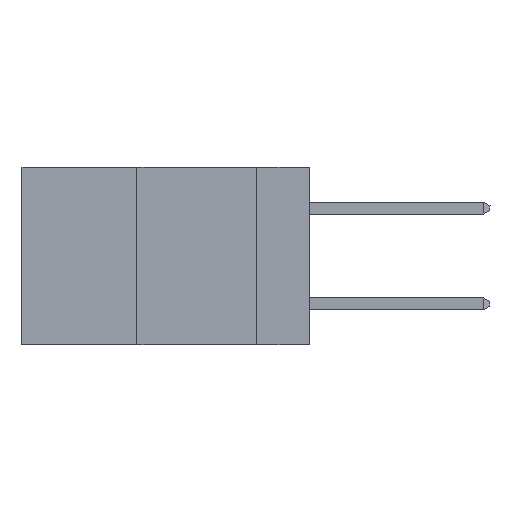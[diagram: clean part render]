
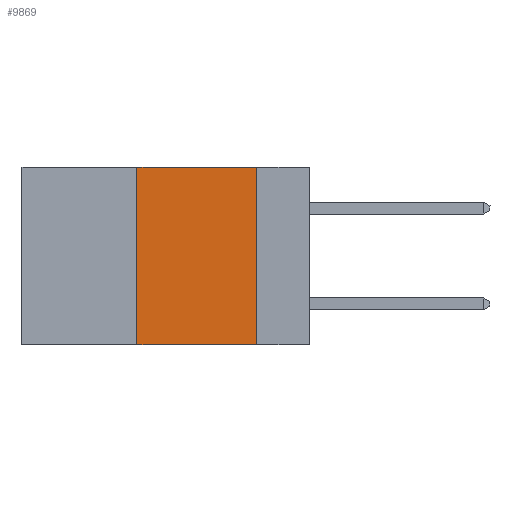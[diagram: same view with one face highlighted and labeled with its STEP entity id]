
A CAD part, left-side view. The second image highlights one B-rep face of the part: STEP entity #9869.
In plain terms, the highlighted planar face has unit normal (-1, 0, 0).
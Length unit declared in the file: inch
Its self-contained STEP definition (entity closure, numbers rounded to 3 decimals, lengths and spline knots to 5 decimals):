
#260 = ORIENTED_EDGE ( 'NONE', *, *, #14562, .F. ) ;
#516 = CARTESIAN_POINT ( 'NONE',  ( 0., 0.6, 0. ) ) ;
#628 = DIRECTION ( 'NONE',  ( 0., 0., -1. ) ) ;
#646 = CARTESIAN_POINT ( 'NONE',  ( 0., 0.36, 0. ) ) ;
#1309 = ORIENTED_EDGE ( 'NONE', *, *, #15781, .F. ) ;
#1714 = LINE ( 'NONE', #516, #2432 ) ;
#1830 = LINE ( 'NONE', #6749, #2767 ) ;
#2074 = EDGE_CURVE ( 'NONE', #8640, #8990, #12546, .T. ) ;
#2318 = CARTESIAN_POINT ( 'NONE',  ( 0., 0.6, -0.37 ) ) ;
#2432 = VECTOR ( 'NONE', #5260, 39.37008 ) ;
#2767 = VECTOR ( 'NONE', #628, 39.37008 ) ;
#2841 = PLANE ( 'NONE',  #9949 ) ;
#2898 = VERTEX_POINT ( 'NONE', #4114 ) ;
#3430 = VERTEX_POINT ( 'NONE', #5232 ) ;
#4091 = ORIENTED_EDGE ( 'NONE', *, *, #12354, .T. ) ;
#4114 = CARTESIAN_POINT ( 'NONE',  ( 0., 0.11, -0.37 ) ) ;
#5232 = CARTESIAN_POINT ( 'NONE',  ( 0., 0.11, 0. ) ) ;
#5260 = DIRECTION ( 'NONE',  ( 0., -1., 0. ) ) ;
#5522 = FACE_OUTER_BOUND ( 'NONE', #11078, .T. ) ;
#5675 = CARTESIAN_POINT ( 'NONE',  ( 0., 0.36, -0.37 ) ) ;
#6749 = CARTESIAN_POINT ( 'NONE',  ( 0., 0.11, 0. ) ) ;
#7774 = DIRECTION ( 'NONE',  ( 1., 0., 0. ) ) ;
#8397 = VECTOR ( 'NONE', #14887, 39.37008 ) ;
#8531 = LINE ( 'NONE', #2318, #8397 ) ;
#8640 = VERTEX_POINT ( 'NONE', #5675 ) ;
#8990 = VERTEX_POINT ( 'NONE', #646 ) ;
#9869 = ADVANCED_FACE ( 'NONE', ( #5522 ), #2841, .F. ) ;
#9949 = AXIS2_PLACEMENT_3D ( 'NONE', #10464, #7774, #12754 ) ;
#10464 = CARTESIAN_POINT ( 'NONE',  ( 0., 0.6, 0. ) ) ;
#11078 = EDGE_LOOP ( 'NONE', ( #260, #1309, #12276, #4091 ) ) ;
#11236 = DIRECTION ( 'NONE',  ( 0., 0., 1. ) ) ;
#12276 = ORIENTED_EDGE ( 'NONE', *, *, #2074, .F. ) ;
#12354 = EDGE_CURVE ( 'NONE', #8640, #2898, #8531, .T. ) ;
#12546 = LINE ( 'NONE', #14233, #15871 ) ;
#12754 = DIRECTION ( 'NONE',  ( 0., 0., -1. ) ) ;
#14233 = CARTESIAN_POINT ( 'NONE',  ( 0., 0.36, 0. ) ) ;
#14562 = EDGE_CURVE ( 'NONE', #3430, #2898, #1830, .T. ) ;
#14887 = DIRECTION ( 'NONE',  ( 0., -1., 0. ) ) ;
#15781 = EDGE_CURVE ( 'NONE', #8990, #3430, #1714, .T. ) ;
#15871 = VECTOR ( 'NONE', #11236, 39.37008 ) ;
